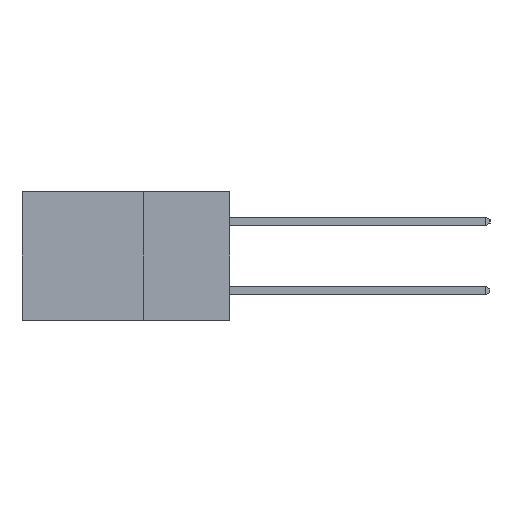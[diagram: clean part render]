
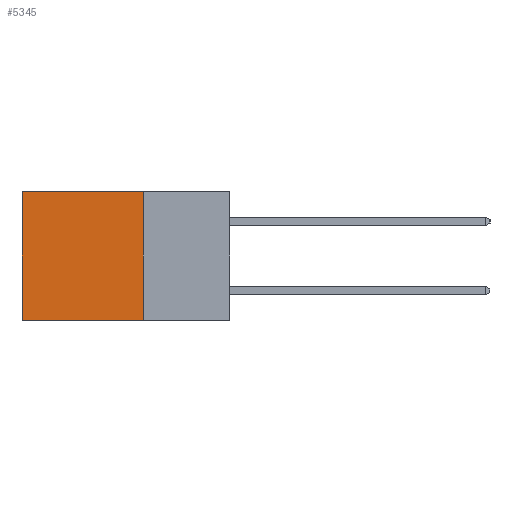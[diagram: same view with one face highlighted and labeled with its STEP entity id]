
A CAD part, left-side view. The second image highlights one B-rep face of the part: STEP entity #5345.
In plain terms, the highlighted planar face has unit normal (-1, 0, 0).
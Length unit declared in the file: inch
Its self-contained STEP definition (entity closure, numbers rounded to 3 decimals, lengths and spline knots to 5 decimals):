
#269 = AXIS2_PLACEMENT_3D ( 'NONE', #4789, #1977, #1853 ) ;
#338 = DIRECTION ( 'NONE',  ( 0., 0., -1. ) ) ;
#1853 = DIRECTION ( 'NONE',  ( 0., 0., -1. ) ) ;
#1977 = DIRECTION ( 'NONE',  ( 1., 0., 0. ) ) ;
#2385 = VECTOR ( 'NONE', #8088, 39.37008 ) ;
#3045 = CARTESIAN_POINT ( 'NONE',  ( 0.298, 0.25, -0.37 ) ) ;
#3339 = ORIENTED_EDGE ( 'NONE', *, *, #13248, .T. ) ;
#3468 = VERTEX_POINT ( 'NONE', #5642 ) ;
#3613 = LINE ( 'NONE', #14425, #14117 ) ;
#4017 = VERTEX_POINT ( 'NONE', #13632 ) ;
#4381 = DIRECTION ( 'NONE',  ( 0., 1., 0. ) ) ;
#4448 = CARTESIAN_POINT ( 'NONE',  ( 0.298, 0.25, 0. ) ) ;
#4670 = PLANE ( 'NONE',  #269 ) ;
#4764 = LINE ( 'NONE', #3045, #14845 ) ;
#4789 = CARTESIAN_POINT ( 'NONE',  ( 0.298, 0.25, 0. ) ) ;
#5345 = ADVANCED_FACE ( 'NONE', ( #8593 ), #4670, .F. ) ;
#5642 = CARTESIAN_POINT ( 'NONE',  ( 0.298, 0.6, 0. ) ) ;
#6505 = DIRECTION ( 'NONE',  ( 0., 1., 0. ) ) ;
#6753 = CARTESIAN_POINT ( 'NONE',  ( 0.298, 0.6, 0. ) ) ;
#6855 = ORIENTED_EDGE ( 'NONE', *, *, #8512, .F. ) ;
#7230 = VERTEX_POINT ( 'NONE', #14668 ) ;
#7269 = ORIENTED_EDGE ( 'NONE', *, *, #10464, .F. ) ;
#8088 = DIRECTION ( 'NONE',  ( 0., 0., -1. ) ) ;
#8512 = EDGE_CURVE ( 'NONE', #9083, #7230, #4764, .T. ) ;
#8593 = FACE_OUTER_BOUND ( 'NONE', #13341, .T. ) ;
#9083 = VERTEX_POINT ( 'NONE', #10949 ) ;
#9536 = EDGE_CURVE ( 'NONE', #4017, #3468, #3613, .T. ) ;
#10464 = EDGE_CURVE ( 'NONE', #4017, #9083, #15897, .T. ) ;
#10949 = CARTESIAN_POINT ( 'NONE',  ( 0.298, 0.25, -0.37 ) ) ;
#12458 = VECTOR ( 'NONE', #338, 39.37008 ) ;
#12949 = LINE ( 'NONE', #6753, #2385 ) ;
#13248 = EDGE_CURVE ( 'NONE', #3468, #7230, #12949, .T. ) ;
#13341 = EDGE_LOOP ( 'NONE', ( #3339, #6855, #7269, #14269 ) ) ;
#13632 = CARTESIAN_POINT ( 'NONE',  ( 0.298, 0.25, 0. ) ) ;
#14117 = VECTOR ( 'NONE', #6505, 39.37008 ) ;
#14269 = ORIENTED_EDGE ( 'NONE', *, *, #9536, .T. ) ;
#14425 = CARTESIAN_POINT ( 'NONE',  ( 0.298, 0.25, 0. ) ) ;
#14668 = CARTESIAN_POINT ( 'NONE',  ( 0.298, 0.6, -0.37 ) ) ;
#14845 = VECTOR ( 'NONE', #4381, 39.37008 ) ;
#15897 = LINE ( 'NONE', #4448, #12458 ) ;
